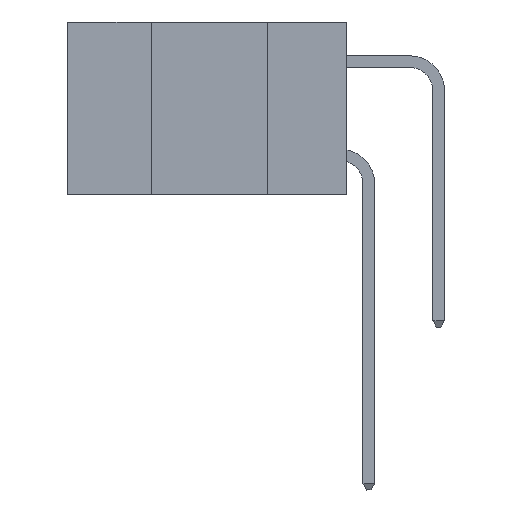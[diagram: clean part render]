
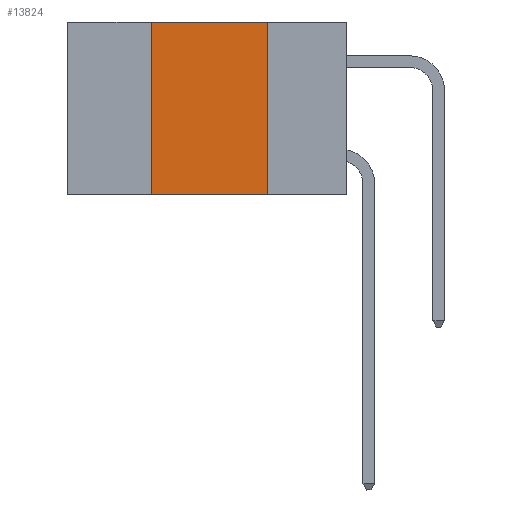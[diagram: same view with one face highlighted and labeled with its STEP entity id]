
A CAD part, left-side view. The second image highlights one B-rep face of the part: STEP entity #13824.
In plain terms, the highlighted planar face has unit normal (-1, 0, 0).
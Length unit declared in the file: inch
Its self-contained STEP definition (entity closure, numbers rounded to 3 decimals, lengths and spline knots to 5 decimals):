
#439 = CARTESIAN_POINT ( 'NONE',  ( 0., 0.42, -0.37 ) ) ;
#559 = CARTESIAN_POINT ( 'NONE',  ( 0., 0.17, 0. ) ) ;
#978 = ORIENTED_EDGE ( 'NONE', *, *, #3651, .F. ) ;
#1024 = EDGE_CURVE ( 'NONE', #3645, #24211, #24720, .T. ) ;
#1979 = DIRECTION ( 'NONE',  ( 0., 0., 1. ) ) ;
#3615 = DIRECTION ( 'NONE',  ( 1., 0., 0. ) ) ;
#3645 = VERTEX_POINT ( 'NONE', #439 ) ;
#3651 = EDGE_CURVE ( 'NONE', #23187, #23359, #17002, .T. ) ;
#4288 = CARTESIAN_POINT ( 'NONE',  ( 0., 0.42, 0. ) ) ;
#4354 = LINE ( 'NONE', #26133, #25245 ) ;
#4897 = CARTESIAN_POINT ( 'NONE',  ( 0., 0.17, -0.37 ) ) ;
#5945 = CARTESIAN_POINT ( 'NONE',  ( 0., 0.42, 0. ) ) ;
#7943 = AXIS2_PLACEMENT_3D ( 'NONE', #9308, #3615, #13671 ) ;
#8883 = EDGE_CURVE ( 'NONE', #3645, #23187, #11929, .T. ) ;
#9014 = EDGE_CURVE ( 'NONE', #23359, #24211, #4354, .T. ) ;
#9308 = CARTESIAN_POINT ( 'NONE',  ( 0., 0.6, 0. ) ) ;
#9512 = ORIENTED_EDGE ( 'NONE', *, *, #9014, .F. ) ;
#10006 = VECTOR ( 'NONE', #16263, 39.37008 ) ;
#10015 = VECTOR ( 'NONE', #1979, 39.37008 ) ;
#10392 = CARTESIAN_POINT ( 'NONE',  ( 0., 0.6, 0. ) ) ;
#11182 = CARTESIAN_POINT ( 'NONE',  ( 0., 0.6, -0.37 ) ) ;
#11929 = LINE ( 'NONE', #5945, #10015 ) ;
#13671 = DIRECTION ( 'NONE',  ( 0., 0., -1. ) ) ;
#13824 = ADVANCED_FACE ( 'NONE', ( #18674 ), #25634, .F. ) ;
#16263 = DIRECTION ( 'NONE',  ( 0., -1., 0. ) ) ;
#17002 = LINE ( 'NONE', #10392, #10006 ) ;
#17667 = DIRECTION ( 'NONE',  ( 0., -1., 0. ) ) ;
#18084 = DIRECTION ( 'NONE',  ( 0., 0., -1. ) ) ;
#18674 = FACE_OUTER_BOUND ( 'NONE', #20246, .T. ) ;
#18983 = ORIENTED_EDGE ( 'NONE', *, *, #8883, .F. ) ;
#20246 = EDGE_LOOP ( 'NONE', ( #9512, #978, #18983, #22917 ) ) ;
#22799 = VECTOR ( 'NONE', #17667, 39.37008 ) ;
#22917 = ORIENTED_EDGE ( 'NONE', *, *, #1024, .T. ) ;
#23187 = VERTEX_POINT ( 'NONE', #4288 ) ;
#23359 = VERTEX_POINT ( 'NONE', #559 ) ;
#24211 = VERTEX_POINT ( 'NONE', #4897 ) ;
#24720 = LINE ( 'NONE', #11182, #22799 ) ;
#25245 = VECTOR ( 'NONE', #18084, 39.37008 ) ;
#25634 = PLANE ( 'NONE',  #7943 ) ;
#26133 = CARTESIAN_POINT ( 'NONE',  ( 0., 0.17, 0. ) ) ;
